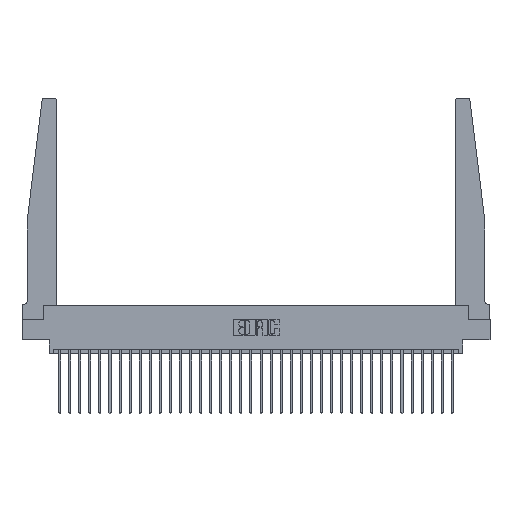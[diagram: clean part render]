
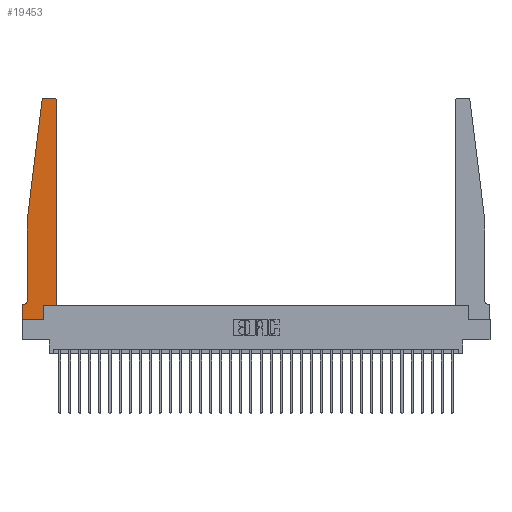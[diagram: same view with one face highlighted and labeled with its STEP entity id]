
A CAD part, top view. The second image highlights one B-rep face of the part: STEP entity #19453.
In plain terms, the highlighted planar face has unit normal (0, 0, 1).
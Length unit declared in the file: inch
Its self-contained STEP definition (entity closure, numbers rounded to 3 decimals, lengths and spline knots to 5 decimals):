
#219 = DIRECTION ( 'NONE',  ( 1., 0., 0. ) ) ;
#310 = DIRECTION ( 'NONE',  ( 1., 0., 0. ) ) ;
#311 = CARTESIAN_POINT ( 'NONE',  ( 0.015, 0.1875, 0.37 ) ) ;
#495 = CARTESIAN_POINT ( 'NONE',  ( 0., 0.1875, 0.37 ) ) ;
#877 = VECTOR ( 'NONE', #22795, 39.37008 ) ;
#914 = LINE ( 'NONE', #23107, #877 ) ;
#1372 = VERTEX_POINT ( 'NONE', #16462 ) ;
#1513 = ORIENTED_EDGE ( 'NONE', *, *, #11054, .T. ) ;
#1846 = VECTOR ( 'NONE', #14636, 39.37008 ) ;
#2458 = CARTESIAN_POINT ( 'NONE',  ( 0.065, 1.25, 0.37 ) ) ;
#2729 = AXIS2_PLACEMENT_3D ( 'NONE', #495, #7432, #24769 ) ;
#3179 = EDGE_CURVE ( 'NONE', #8719, #20428, #5616, .T. ) ;
#3210 = EDGE_CURVE ( 'NONE', #12004, #20495, #14660, .T. ) ;
#3510 = ORIENTED_EDGE ( 'NONE', *, *, #16936, .T. ) ;
#3871 = AXIS2_PLACEMENT_3D ( 'NONE', #19773, #4992, #12677 ) ;
#4049 = LINE ( 'NONE', #14006, #11898 ) ;
#4453 = EDGE_CURVE ( 'NONE', #21908, #4729, #4524, .T. ) ;
#4524 = LINE ( 'NONE', #21886, #1846 ) ;
#4649 = DIRECTION ( 'NONE',  ( -1., 0., 0. ) ) ;
#4729 = VERTEX_POINT ( 'NONE', #25691 ) ;
#4902 = CARTESIAN_POINT ( 'NONE',  ( 0.2605, 0.18, 0.37 ) ) ;
#4992 = DIRECTION ( 'NONE',  ( 0., 0., 1. ) ) ;
#5068 = CARTESIAN_POINT ( 'NONE',  ( 0.425, 2.72, 0.37 ) ) ;
#5447 = DIRECTION ( 'NONE',  ( -0.122, -0.992, 0. ) ) ;
#5616 = LINE ( 'NONE', #10591, #12584 ) ;
#5709 = VECTOR ( 'NONE', #219, 39.37008 ) ;
#5928 = LINE ( 'NONE', #27458, #9913 ) ;
#6579 = CARTESIAN_POINT ( 'NONE',  ( 0.015, 0.2375, 0.37 ) ) ;
#6962 = EDGE_CURVE ( 'NONE', #20495, #1372, #11283, .T. ) ;
#7385 = CARTESIAN_POINT ( 'NONE',  ( 0.27653, 2.72, 0.37 ) ) ;
#7432 = DIRECTION ( 'NONE',  ( 0., 0., 1. ) ) ;
#7564 = DIRECTION ( 'NONE',  ( 0., -1., 0. ) ) ;
#7653 = ORIENTED_EDGE ( 'NONE', *, *, #6962, .T. ) ;
#7939 = LINE ( 'NONE', #24506, #5709 ) ;
#7971 = ORIENTED_EDGE ( 'NONE', *, *, #31613, .T. ) ;
#8719 = VERTEX_POINT ( 'NONE', #4902 ) ;
#9280 = ORIENTED_EDGE ( 'NONE', *, *, #29341, .T. ) ;
#9913 = VECTOR ( 'NONE', #5447, 39.37008 ) ;
#10148 = FACE_OUTER_BOUND ( 'NONE', #22002, .T. ) ;
#10265 = VERTEX_POINT ( 'NONE', #18258 ) ;
#10591 = CARTESIAN_POINT ( 'NONE',  ( 0.425, 0.18, 0.37 ) ) ;
#11054 = EDGE_CURVE ( 'NONE', #4729, #28453, #29569, .T. ) ;
#11283 = LINE ( 'NONE', #21099, #26019 ) ;
#11839 = CARTESIAN_POINT ( 'NONE',  ( 0.2605, 0.18, 0.37 ) ) ;
#11898 = VECTOR ( 'NONE', #13848, 39.37008 ) ;
#12004 = VERTEX_POINT ( 'NONE', #5068 ) ;
#12584 = VECTOR ( 'NONE', #310, 39.37008 ) ;
#12677 = DIRECTION ( 'NONE',  ( 1., 0., 0. ) ) ;
#13743 = VECTOR ( 'NONE', #26466, 39.37008 ) ;
#13761 = EDGE_CURVE ( 'NONE', #20052, #21908, #30656, .T. ) ;
#13848 = DIRECTION ( 'NONE',  ( 0., -1., 0. ) ) ;
#14006 = CARTESIAN_POINT ( 'NONE',  ( 0.065, 1.25, 0.37 ) ) ;
#14057 = EDGE_CURVE ( 'NONE', #20428, #12004, #914, .T. ) ;
#14636 = DIRECTION ( 'NONE',  ( -1., 0., 0. ) ) ;
#14660 = CIRCLE ( 'NONE', #3871, 0.03 ) ;
#15081 = CARTESIAN_POINT ( 'NONE',  ( 0.065, 0.2375, 0.37 ) ) ;
#15544 = ORIENTED_EDGE ( 'NONE', *, *, #18132, .T. ) ;
#16288 = ORIENTED_EDGE ( 'NONE', *, *, #3210, .T. ) ;
#16462 = CARTESIAN_POINT ( 'NONE',  ( 0.27653, 2.75, 0.37 ) ) ;
#16529 = EDGE_CURVE ( 'NONE', #10265, #8719, #21502, .T. ) ;
#16936 = EDGE_CURVE ( 'NONE', #1372, #31491, #23653, .T. ) ;
#16948 = ORIENTED_EDGE ( 'NONE', *, *, #4453, .T. ) ;
#17450 = ORIENTED_EDGE ( 'NONE', *, *, #3179, .T. ) ;
#17843 = ORIENTED_EDGE ( 'NONE', *, *, #13761, .T. ) ;
#18132 = EDGE_CURVE ( 'NONE', #31062, #20052, #4049, .T. ) ;
#18258 = CARTESIAN_POINT ( 'NONE',  ( 0.2605, 0., 0.37 ) ) ;
#19151 = CARTESIAN_POINT ( 'NONE',  ( 0.425, 0.18, 0.37 ) ) ;
#19453 = ADVANCED_FACE ( 'NONE', ( #10148 ), #31681, .T. ) ;
#19773 = CARTESIAN_POINT ( 'NONE',  ( 0.395, 2.72, 0.37 ) ) ;
#20052 = VERTEX_POINT ( 'NONE', #15081 ) ;
#20236 = CARTESIAN_POINT ( 'NONE',  ( 0.24675, 2.72367, 0.37 ) ) ;
#20428 = VERTEX_POINT ( 'NONE', #19151 ) ;
#20495 = VERTEX_POINT ( 'NONE', #26855 ) ;
#21099 = CARTESIAN_POINT ( 'NONE',  ( 0.25, 2.75, 0.37 ) ) ;
#21502 = LINE ( 'NONE', #11839, #13743 ) ;
#21886 = CARTESIAN_POINT ( 'NONE',  ( 0.065, 0.1875, 0.37 ) ) ;
#21908 = VERTEX_POINT ( 'NONE', #311 ) ;
#22002 = EDGE_LOOP ( 'NONE', ( #7653, #3510, #7971, #15544, #17843, #16948, #1513, #9280, #24806, #17450, #27084, #16288 ) ) ;
#22795 = DIRECTION ( 'NONE',  ( 0., 1., 0. ) ) ;
#23107 = CARTESIAN_POINT ( 'NONE',  ( 0.425, 0.18, 0.37 ) ) ;
#23462 = AXIS2_PLACEMENT_3D ( 'NONE', #6579, #23941, #4649 ) ;
#23653 = CIRCLE ( 'NONE', #26209, 0.03 ) ;
#23941 = DIRECTION ( 'NONE',  ( 0., 0., -1. ) ) ;
#24506 = CARTESIAN_POINT ( 'NONE',  ( 0., 0., 0.37 ) ) ;
#24769 = DIRECTION ( 'NONE',  ( 1., 0., 0. ) ) ;
#24806 = ORIENTED_EDGE ( 'NONE', *, *, #16529, .T. ) ;
#24893 = CARTESIAN_POINT ( 'NONE',  ( 0., 0., 0.37 ) ) ;
#25691 = CARTESIAN_POINT ( 'NONE',  ( 0., 0.1875, 0.37 ) ) ;
#26019 = VECTOR ( 'NONE', #30895, 39.37008 ) ;
#26209 = AXIS2_PLACEMENT_3D ( 'NONE', #7385, #31631, #29227 ) ;
#26415 = VECTOR ( 'NONE', #7564, 39.37008 ) ;
#26466 = DIRECTION ( 'NONE',  ( 0., 1., 0. ) ) ;
#26855 = CARTESIAN_POINT ( 'NONE',  ( 0.395, 2.75, 0.37 ) ) ;
#27084 = ORIENTED_EDGE ( 'NONE', *, *, #14057, .T. ) ;
#27458 = CARTESIAN_POINT ( 'NONE',  ( 0.065, 1.25, 0.37 ) ) ;
#28453 = VERTEX_POINT ( 'NONE', #30248 ) ;
#29227 = DIRECTION ( 'NONE',  ( 1., 0., 0. ) ) ;
#29341 = EDGE_CURVE ( 'NONE', #28453, #10265, #7939, .T. ) ;
#29569 = LINE ( 'NONE', #24893, #26415 ) ;
#30248 = CARTESIAN_POINT ( 'NONE',  ( 0., 0., 0.37 ) ) ;
#30656 = CIRCLE ( 'NONE', #23462, 0.05 ) ;
#30895 = DIRECTION ( 'NONE',  ( -1., 0., 0. ) ) ;
#31062 = VERTEX_POINT ( 'NONE', #2458 ) ;
#31491 = VERTEX_POINT ( 'NONE', #20236 ) ;
#31613 = EDGE_CURVE ( 'NONE', #31491, #31062, #5928, .T. ) ;
#31631 = DIRECTION ( 'NONE',  ( 0., 0., 1. ) ) ;
#31681 = PLANE ( 'NONE',  #2729 ) ;
